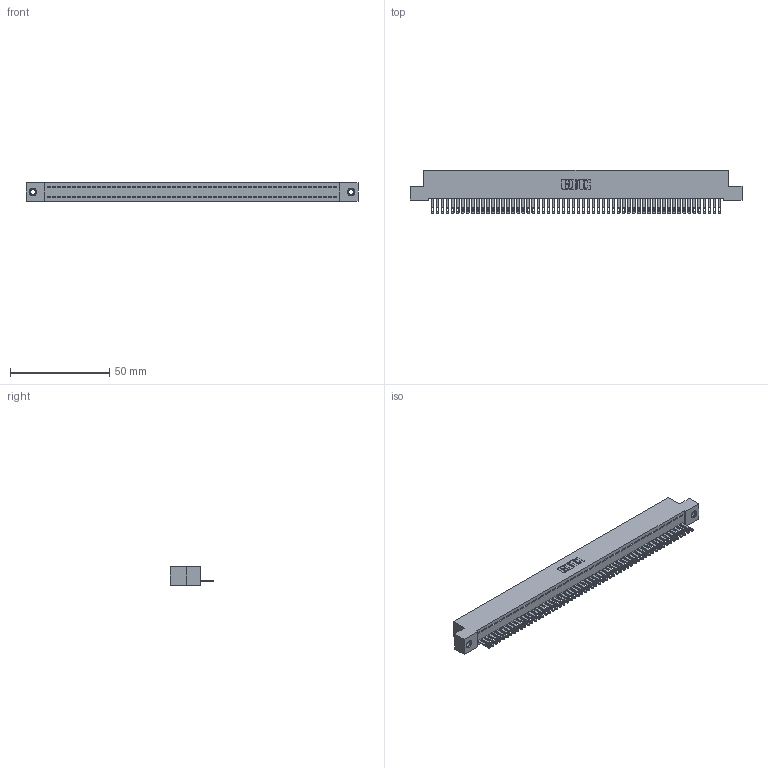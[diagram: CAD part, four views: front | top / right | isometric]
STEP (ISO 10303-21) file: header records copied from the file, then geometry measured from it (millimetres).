
FILE_DESCRIPTION (( 'STEP AP203' ), '1' );
FILE_NAME ('892-058-500-107.STEP', '2020-09-21T18:58:10', ( '' ), ( '' ), 'SwSTEP 2.0', 'SolidWorks 2020', '' );
FILE_SCHEMA (( 'CONFIG_CONTROL_DESIGN' ));
Length unit declared in the file: inch
Products named in the file (4): 892-058-500-107; 842 Part_TI; 345-292-001_345-293-100; 345-250-001_345-250-005-103
Assembly tree (61 placements, depth 2):
  892-058-500-107
    842 Part_TI
    345-292-001_345-293-100  x58
    345-250-001_345-250-005-103  x2
Bounding box: 167.64 x 21.85 x 9.4 mm (x, y, z)
Volume: 14780.8 mm3; surface area: 22150.1 mm2
Topology: 61 solids, 61 shells, 3302 faces, 10179 edges, 6778 vertices
Faces by surface type: plane 2186, cylinder 1100, cone 12, torus 4
Entity records: 34372 total; most frequent: CARTESIAN_POINT 5907, ORIENTED_EDGE 5894, DIRECTION 4985, EDGE_CURVE 2947, LINE 2795, VECTOR 2795, VERTEX_POINT 1960, AXIS2_PLACEMENT_3D 1095
